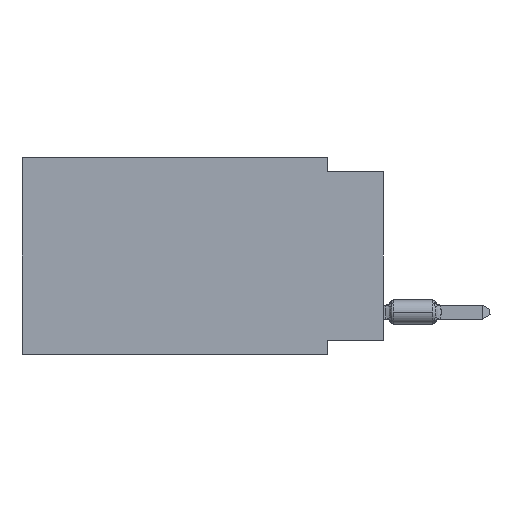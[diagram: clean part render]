
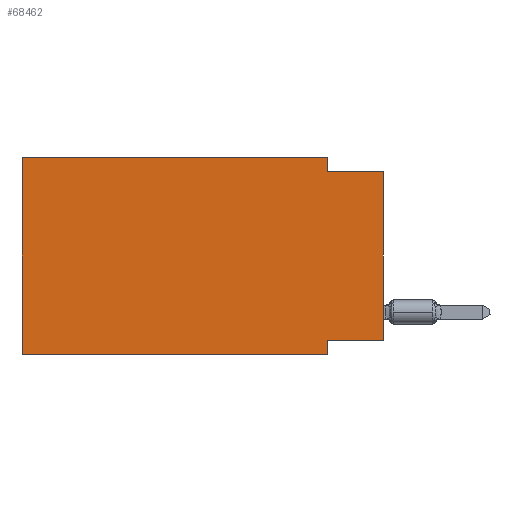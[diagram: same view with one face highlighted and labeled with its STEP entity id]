
A CAD part, left-side view. The second image highlights one B-rep face of the part: STEP entity #68462.
In plain terms, the highlighted planar face has unit normal (-1, 0, 0).
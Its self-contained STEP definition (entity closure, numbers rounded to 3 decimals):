
#644 = EDGE_CURVE ( 'NONE', #22383, #29503, #29275, .T. ) ;
#694 = ORIENTED_EDGE ( 'NONE', *, *, #90759, .F. ) ;
#3650 = LINE ( 'NONE', #10728, #32542 ) ;
#4014 = CARTESIAN_POINT ( 'NONE',  ( 0., 16.383, 0. ) ) ;
#5002 = ORIENTED_EDGE ( 'NONE', *, *, #644, .T. ) ;
#6891 = VERTEX_POINT ( 'NONE', #26863 ) ;
#8300 = ORIENTED_EDGE ( 'NONE', *, *, #29641, .F. ) ;
#8604 = EDGE_CURVE ( 'NONE', #60237, #83243, #27775, .T. ) ;
#10728 = CARTESIAN_POINT ( 'NONE',  ( 0., 2.54, -8.89 ) ) ;
#10928 = CARTESIAN_POINT ( 'NONE',  ( 0., 2.54, 0. ) ) ;
#11058 = DIRECTION ( 'NONE',  ( 0., 0., -1. ) ) ;
#12064 = PLANE ( 'NONE',  #16108 ) ;
#13722 = ORIENTED_EDGE ( 'NONE', *, *, #83347, .F. ) ;
#16108 = AXIS2_PLACEMENT_3D ( 'NONE', #4014, #74018, #11058 ) ;
#17453 = CARTESIAN_POINT ( 'NONE',  ( 0., 0., -8.255 ) ) ;
#17901 = CARTESIAN_POINT ( 'NONE',  ( 0., 16.383, 0. ) ) ;
#21705 = CARTESIAN_POINT ( 'NONE',  ( 0., 0., 0. ) ) ;
#22383 = VERTEX_POINT ( 'NONE', #17453 ) ;
#26863 = CARTESIAN_POINT ( 'NONE',  ( 0., 16.383, -8.89 ) ) ;
#27775 = LINE ( 'NONE', #67552, #68073 ) ;
#29275 = LINE ( 'NONE', #21705, #60835 ) ;
#29503 = VERTEX_POINT ( 'NONE', #90338 ) ;
#29641 = EDGE_CURVE ( 'NONE', #83243, #44304, #59125, .T. ) ;
#30993 = VERTEX_POINT ( 'NONE', #35337 ) ;
#32542 = VECTOR ( 'NONE', #94357, 1000. ) ;
#33100 = LINE ( 'NONE', #63831, #53933 ) ;
#35337 = CARTESIAN_POINT ( 'NONE',  ( 0., 2.54, -8.255 ) ) ;
#35967 = VECTOR ( 'NONE', #64273, 1000. ) ;
#40993 = ORIENTED_EDGE ( 'NONE', *, *, #42683, .T. ) ;
#41163 = DIRECTION ( 'NONE',  ( 0., 1., 0. ) ) ;
#42040 = ORIENTED_EDGE ( 'NONE', *, *, #45109, .F. ) ;
#42683 = EDGE_CURVE ( 'NONE', #6891, #60435, #82760, .T. ) ;
#44304 = VERTEX_POINT ( 'NONE', #73104 ) ;
#45109 = EDGE_CURVE ( 'NONE', #22383, #30993, #33100, .T. ) ;
#45469 = DIRECTION ( 'NONE',  ( 0., -1., 0. ) ) ;
#51562 = DIRECTION ( 'NONE',  ( 0., 0., -1. ) ) ;
#53933 = VECTOR ( 'NONE', #41163, 1000. ) ;
#59125 = LINE ( 'NONE', #89837, #89262 ) ;
#59289 = DIRECTION ( 'NONE',  ( 0., -1., 0. ) ) ;
#60237 = VERTEX_POINT ( 'NONE', #63573 ) ;
#60435 = VERTEX_POINT ( 'NONE', #89719 ) ;
#60579 = VECTOR ( 'NONE', #59289, 1000. ) ;
#60731 = EDGE_CURVE ( 'NONE', #30993, #60435, #3650, .T. ) ;
#60835 = VECTOR ( 'NONE', #83166, 1000. ) ;
#61081 = CARTESIAN_POINT ( 'NONE',  ( 0., 16.383, -8.89 ) ) ;
#62769 = EDGE_LOOP ( 'NONE', ( #5002, #13722, #8300, #88460, #694, #40993, #97045, #42040 ) ) ;
#63573 = CARTESIAN_POINT ( 'NONE',  ( 0., 16.383, 0. ) ) ;
#63831 = CARTESIAN_POINT ( 'NONE',  ( 0., 0., -8.255 ) ) ;
#64273 = DIRECTION ( 'NONE',  ( 0., 0., 1. ) ) ;
#67552 = CARTESIAN_POINT ( 'NONE',  ( 0., 16.383, 0. ) ) ;
#68073 = VECTOR ( 'NONE', #97777, 1000. ) ;
#68462 = ADVANCED_FACE ( 'NONE', ( #81074 ), #12064, .F. ) ;
#68818 = LINE ( 'NONE', #82429, #60579 ) ;
#73104 = CARTESIAN_POINT ( 'NONE',  ( 0., 2.54, -0.635 ) ) ;
#74018 = DIRECTION ( 'NONE',  ( 1., 0., 0. ) ) ;
#74490 = VECTOR ( 'NONE', #45469, 1000. ) ;
#81074 = FACE_OUTER_BOUND ( 'NONE', #62769, .T. ) ;
#82429 = CARTESIAN_POINT ( 'NONE',  ( 0., 0., -0.635 ) ) ;
#82760 = LINE ( 'NONE', #61081, #74490 ) ;
#83166 = DIRECTION ( 'NONE',  ( 0., 0., 1. ) ) ;
#83243 = VERTEX_POINT ( 'NONE', #10928 ) ;
#83347 = EDGE_CURVE ( 'NONE', #44304, #29503, #68818, .T. ) ;
#88460 = ORIENTED_EDGE ( 'NONE', *, *, #8604, .F. ) ;
#89262 = VECTOR ( 'NONE', #51562, 1000. ) ;
#89719 = CARTESIAN_POINT ( 'NONE',  ( 0., 2.54, -8.89 ) ) ;
#89837 = CARTESIAN_POINT ( 'NONE',  ( 0., 2.54, 0. ) ) ;
#90338 = CARTESIAN_POINT ( 'NONE',  ( 0., 0., -0.635 ) ) ;
#90759 = EDGE_CURVE ( 'NONE', #6891, #60237, #95979, .T. ) ;
#94357 = DIRECTION ( 'NONE',  ( 0., 0., -1. ) ) ;
#95979 = LINE ( 'NONE', #17901, #35967 ) ;
#97045 = ORIENTED_EDGE ( 'NONE', *, *, #60731, .F. ) ;
#97777 = DIRECTION ( 'NONE',  ( 0., -1., 0. ) ) ;
